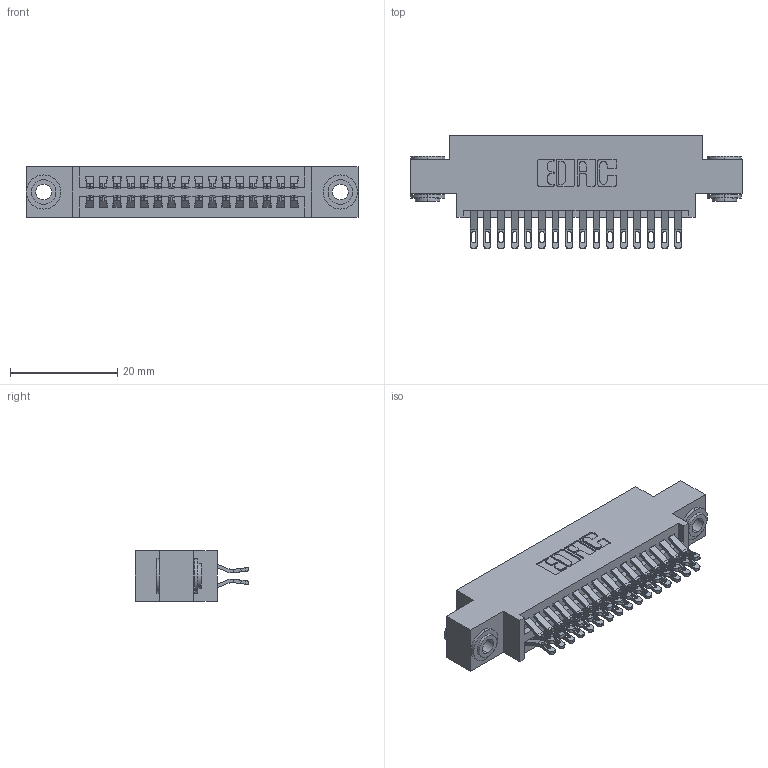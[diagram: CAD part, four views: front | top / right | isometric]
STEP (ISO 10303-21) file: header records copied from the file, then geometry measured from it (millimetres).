
FILE_DESCRIPTION (( 'STEP AP203' ), '1' );
FILE_NAME ('395-032-555-803.STEP', '2018-11-12T22:34:42', ( '' ), ( '' ), 'SwSTEP 2.0', 'SolidWorks 2016', '' );
FILE_SCHEMA (( 'CONFIG_CONTROL_DESIGN' ));
Length unit declared in the file: inch
Products named in the file (4): 345-292-001_555 Tail; 395-032-555-803; 345-250-002_345-250-002-102; 345 Part_0.170 Offset - 0.156 Dia-TH
Assembly tree (35 placements, depth 2):
  395-032-555-803
    345 Part_0.170 Offset - 0.156 Dia-TH
    345-292-001_555 Tail  x32
    345-250-002_345-250-002-102  x2
Bounding box: 61.85 x 21.13 x 9.4 mm (x, y, z)
Volume: 5765.6 mm3; surface area: 8690.1 mm2
Topology: 35 solids, 35 shells, 1960 faces, 6093 edges, 4058 vertices
Faces by surface type: plane 1086, cylinder 866, cone 8
Entity records: 17162 total; most frequent: CARTESIAN_POINT 2913, ORIENTED_EDGE 2810, DIRECTION 2599, EDGE_CURVE 1405, VECTOR 1165, LINE 1165, VERTEX_POINT 934, AXIS2_PLACEMENT_3D 717
